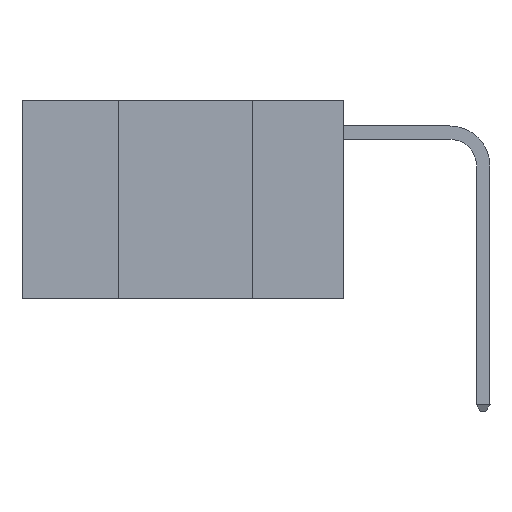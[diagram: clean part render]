
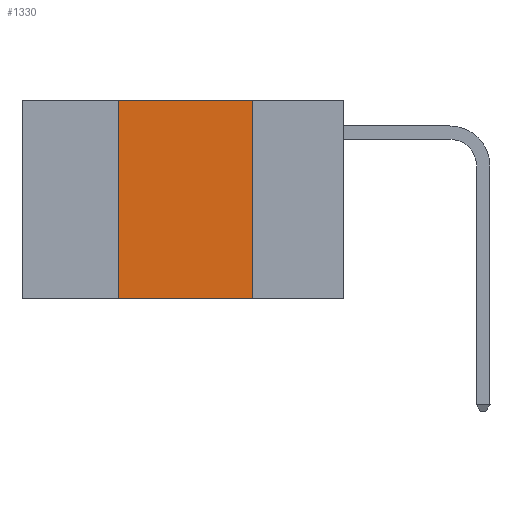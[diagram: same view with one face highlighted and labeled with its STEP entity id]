
A CAD part, left-side view. The second image highlights one B-rep face of the part: STEP entity #1330.
In plain terms, the highlighted planar face has unit normal (-1, 0, 0).
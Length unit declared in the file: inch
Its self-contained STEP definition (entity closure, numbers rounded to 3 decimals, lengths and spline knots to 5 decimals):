
#258 = CARTESIAN_POINT ( 'NONE',  ( 0., 0.42, 0. ) ) ;
#387 = CARTESIAN_POINT ( 'NONE',  ( 0., 0.17, 0. ) ) ;
#885 = CARTESIAN_POINT ( 'NONE',  ( 0., 0.6, -0.37 ) ) ;
#1035 = EDGE_CURVE ( 'NONE', #9845, #6984, #12858, .T. ) ;
#1330 = ADVANCED_FACE ( 'NONE', ( #12439 ), #10097, .F. ) ;
#1386 = LINE ( 'NONE', #12674, #8601 ) ;
#1851 = VECTOR ( 'NONE', #5272, 39.37008 ) ;
#2554 = CARTESIAN_POINT ( 'NONE',  ( 0., 0.6, 0. ) ) ;
#3060 = CARTESIAN_POINT ( 'NONE',  ( 0., 0.42, 0. ) ) ;
#3945 = ORIENTED_EDGE ( 'NONE', *, *, #4241, .F. ) ;
#4241 = EDGE_CURVE ( 'NONE', #6984, #14262, #1386, .T. ) ;
#5213 = LINE ( 'NONE', #3060, #1851 ) ;
#5272 = DIRECTION ( 'NONE',  ( 0., 0., 1. ) ) ;
#5392 = DIRECTION ( 'NONE',  ( 0., -1., 0. ) ) ;
#5731 = DIRECTION ( 'NONE',  ( 0., 0., -1. ) ) ;
#6909 = DIRECTION ( 'NONE',  ( 1., 0., 0. ) ) ;
#6945 = ORIENTED_EDGE ( 'NONE', *, *, #1035, .F. ) ;
#6984 = VERTEX_POINT ( 'NONE', #387 ) ;
#7108 = DIRECTION ( 'NONE',  ( 0., -1., 0. ) ) ;
#7203 = EDGE_CURVE ( 'NONE', #10665, #14262, #11008, .T. ) ;
#8490 = VECTOR ( 'NONE', #5392, 39.37008 ) ;
#8601 = VECTOR ( 'NONE', #5731, 39.37008 ) ;
#9339 = ORIENTED_EDGE ( 'NONE', *, *, #14212, .F. ) ;
#9543 = AXIS2_PLACEMENT_3D ( 'NONE', #10236, #6909, #11424 ) ;
#9845 = VERTEX_POINT ( 'NONE', #258 ) ;
#10097 = PLANE ( 'NONE',  #9543 ) ;
#10225 = VECTOR ( 'NONE', #7108, 39.37008 ) ;
#10236 = CARTESIAN_POINT ( 'NONE',  ( 0., 0.6, 0. ) ) ;
#10665 = VERTEX_POINT ( 'NONE', #12746 ) ;
#11008 = LINE ( 'NONE', #885, #8490 ) ;
#11424 = DIRECTION ( 'NONE',  ( 0., 0., -1. ) ) ;
#12439 = FACE_OUTER_BOUND ( 'NONE', #14447, .T. ) ;
#12643 = ORIENTED_EDGE ( 'NONE', *, *, #7203, .T. ) ;
#12674 = CARTESIAN_POINT ( 'NONE',  ( 0., 0.17, 0. ) ) ;
#12746 = CARTESIAN_POINT ( 'NONE',  ( 0., 0.42, -0.37 ) ) ;
#12858 = LINE ( 'NONE', #2554, #10225 ) ;
#14212 = EDGE_CURVE ( 'NONE', #10665, #9845, #5213, .T. ) ;
#14262 = VERTEX_POINT ( 'NONE', #14331 ) ;
#14331 = CARTESIAN_POINT ( 'NONE',  ( 0., 0.17, -0.37 ) ) ;
#14447 = EDGE_LOOP ( 'NONE', ( #3945, #6945, #9339, #12643 ) ) ;
